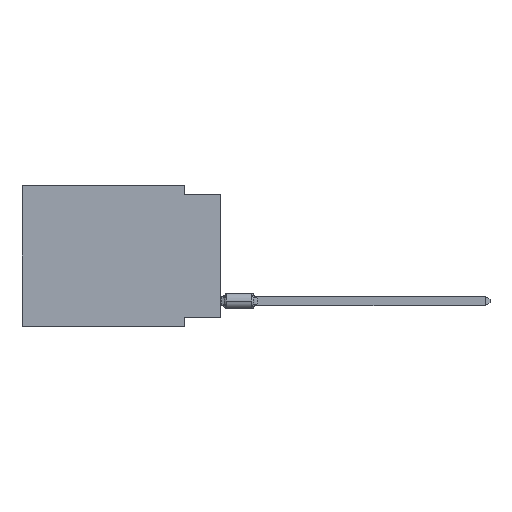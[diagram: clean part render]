
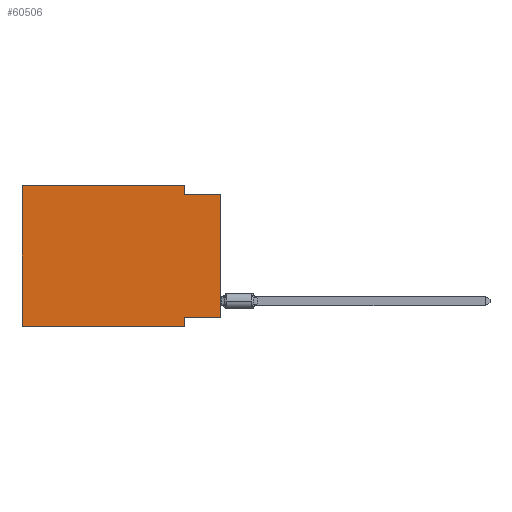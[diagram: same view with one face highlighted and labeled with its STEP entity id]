
A CAD part, left-side view. The second image highlights one B-rep face of the part: STEP entity #60506.
In plain terms, the highlighted planar face has unit normal (-1, 0, 0).
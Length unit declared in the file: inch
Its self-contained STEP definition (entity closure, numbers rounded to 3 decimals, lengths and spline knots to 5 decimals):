
#10 = LINE ( 'NONE', #61957, #57553 ) ;
#34 = AXIS2_PLACEMENT_3D ( 'NONE', #27451, #16596, #60825 ) ;
#2801 = VECTOR ( 'NONE', #41496, 39.37008 ) ;
#6198 = CARTESIAN_POINT ( 'NONE',  ( 0., 0.1, -0.365 ) ) ;
#6859 = DIRECTION ( 'NONE',  ( 0., 0., 1. ) ) ;
#7503 = ORIENTED_EDGE ( 'NONE', *, *, #59413, .F. ) ;
#8282 = CARTESIAN_POINT ( 'NONE',  ( 0., 0., -0.025 ) ) ;
#8596 = EDGE_CURVE ( 'NONE', #38815, #50796, #48998, .T. ) ;
#8773 = VECTOR ( 'NONE', #9221, 39.37008 ) ;
#9221 = DIRECTION ( 'NONE',  ( 0., 1., 0. ) ) ;
#10290 = CARTESIAN_POINT ( 'NONE',  ( 0., 0., -0.365 ) ) ;
#14410 = DIRECTION ( 'NONE',  ( 0., 0., -1. ) ) ;
#15065 = EDGE_CURVE ( 'NONE', #63108, #61980, #10, .T. ) ;
#15261 = CARTESIAN_POINT ( 'NONE',  ( 0., 0.55, -0.39 ) ) ;
#16596 = DIRECTION ( 'NONE',  ( 1., 0., 0. ) ) ;
#18912 = ORIENTED_EDGE ( 'NONE', *, *, #35508, .F. ) ;
#19238 = CARTESIAN_POINT ( 'NONE',  ( 0., 0.55, 0. ) ) ;
#19866 = CARTESIAN_POINT ( 'NONE',  ( 0., 0., -0.365 ) ) ;
#21847 = CARTESIAN_POINT ( 'NONE',  ( 0., 0.55, -0.39 ) ) ;
#21855 = VECTOR ( 'NONE', #14410, 39.37008 ) ;
#24059 = ORIENTED_EDGE ( 'NONE', *, *, #8596, .T. ) ;
#27451 = CARTESIAN_POINT ( 'NONE',  ( 0., 0.55, 0. ) ) ;
#28754 = DIRECTION ( 'NONE',  ( 0., 0., -1. ) ) ;
#29462 = CARTESIAN_POINT ( 'NONE',  ( 0., 0.1, -0.39 ) ) ;
#29684 = EDGE_CURVE ( 'NONE', #38815, #30001, #52973, .T. ) ;
#30001 = VERTEX_POINT ( 'NONE', #56191 ) ;
#32098 = VERTEX_POINT ( 'NONE', #35872 ) ;
#32811 = EDGE_LOOP ( 'NONE', ( #41124, #37907, #35185, #7503, #60397, #24059, #18912, #40957 ) ) ;
#33088 = CARTESIAN_POINT ( 'NONE',  ( 0., 0.1, -0.025 ) ) ;
#34315 = CARTESIAN_POINT ( 'NONE',  ( 0., 0.55, 0. ) ) ;
#35185 = ORIENTED_EDGE ( 'NONE', *, *, #49240, .F. ) ;
#35508 = EDGE_CURVE ( 'NONE', #40554, #50796, #56700, .T. ) ;
#35872 = CARTESIAN_POINT ( 'NONE',  ( 0., 0.1, 0. ) ) ;
#37907 = ORIENTED_EDGE ( 'NONE', *, *, #41616, .F. ) ;
#38284 = VECTOR ( 'NONE', #61879, 39.37008 ) ;
#38815 = VERTEX_POINT ( 'NONE', #21847 ) ;
#39845 = LINE ( 'NONE', #47050, #21855 ) ;
#40554 = VERTEX_POINT ( 'NONE', #6198 ) ;
#40957 = ORIENTED_EDGE ( 'NONE', *, *, #45400, .F. ) ;
#41124 = ORIENTED_EDGE ( 'NONE', *, *, #15065, .T. ) ;
#41496 = DIRECTION ( 'NONE',  ( 0., -1., 0. ) ) ;
#41616 = EDGE_CURVE ( 'NONE', #42634, #61980, #43554, .T. ) ;
#42634 = VERTEX_POINT ( 'NONE', #33088 ) ;
#43554 = LINE ( 'NONE', #47667, #2801 ) ;
#44847 = LINE ( 'NONE', #34315, #38284 ) ;
#45400 = EDGE_CURVE ( 'NONE', #63108, #40554, #58894, .T. ) ;
#45954 = CARTESIAN_POINT ( 'NONE',  ( 0., 0.1, -0.39 ) ) ;
#46387 = VECTOR ( 'NONE', #64551, 39.37008 ) ;
#47050 = CARTESIAN_POINT ( 'NONE',  ( 0., 0.1, 0. ) ) ;
#47352 = VECTOR ( 'NONE', #54437, 39.37008 ) ;
#47667 = CARTESIAN_POINT ( 'NONE',  ( 0., 0., -0.025 ) ) ;
#48998 = LINE ( 'NONE', #15261, #47352 ) ;
#49118 = VECTOR ( 'NONE', #28754, 39.37008 ) ;
#49240 = EDGE_CURVE ( 'NONE', #32098, #42634, #39845, .T. ) ;
#50796 = VERTEX_POINT ( 'NONE', #45954 ) ;
#52973 = LINE ( 'NONE', #19238, #46387 ) ;
#54437 = DIRECTION ( 'NONE',  ( 0., -1., 0. ) ) ;
#56191 = CARTESIAN_POINT ( 'NONE',  ( 0., 0.55, 0. ) ) ;
#56700 = LINE ( 'NONE', #29462, #49118 ) ;
#57553 = VECTOR ( 'NONE', #6859, 39.37008 ) ;
#58894 = LINE ( 'NONE', #10290, #8773 ) ;
#59413 = EDGE_CURVE ( 'NONE', #30001, #32098, #44847, .T. ) ;
#60120 = PLANE ( 'NONE',  #34 ) ;
#60397 = ORIENTED_EDGE ( 'NONE', *, *, #29684, .F. ) ;
#60480 = FACE_OUTER_BOUND ( 'NONE', #32811, .T. ) ;
#60506 = ADVANCED_FACE ( 'NONE', ( #60480 ), #60120, .F. ) ;
#60825 = DIRECTION ( 'NONE',  ( 0., 0., -1. ) ) ;
#61879 = DIRECTION ( 'NONE',  ( 0., -1., 0. ) ) ;
#61957 = CARTESIAN_POINT ( 'NONE',  ( 0., 0., 0. ) ) ;
#61980 = VERTEX_POINT ( 'NONE', #8282 ) ;
#63108 = VERTEX_POINT ( 'NONE', #19866 ) ;
#64551 = DIRECTION ( 'NONE',  ( 0., 0., 1. ) ) ;
